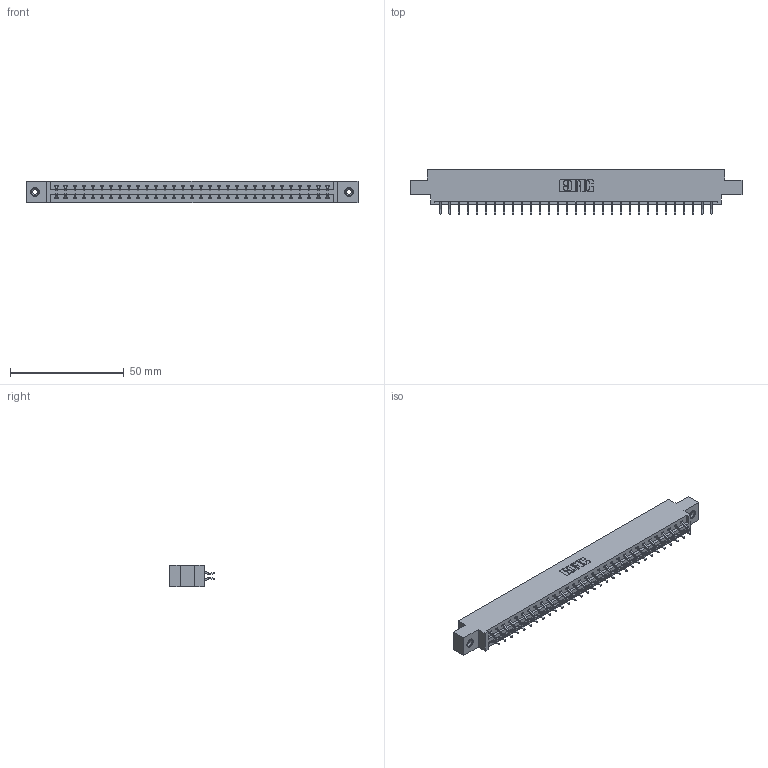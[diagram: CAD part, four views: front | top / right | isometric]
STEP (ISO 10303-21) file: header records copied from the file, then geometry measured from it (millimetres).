
FILE_DESCRIPTION (( 'STEP AP203' ), '1' );
FILE_NAME ('387-062-556-808.STEP', '2018-09-21T06:06:02', ( '' ), ( '' ), 'SwSTEP 2.0', 'SolidWorks 2016', '' );
FILE_SCHEMA (( 'CONFIG_CONTROL_DESIGN' ));
Length unit declared in the file: inch
Products named in the file (4): 345-250-001_345-250-003-102; 387-062-556-808; 337 Part_0.170 Offset - 0.156 Dia-TI; 345-292-001_556 Tail
Assembly tree (65 placements, depth 2):
  387-062-556-808
    337 Part_0.170 Offset - 0.156 Dia-TI
    345-292-001_556 Tail  x62
    345-250-001_345-250-003-102  x2
Bounding box: 145.85 x 19.57 x 9.4 mm (x, y, z)
Volume: 15097.6 mm3; surface area: 17027.4 mm2
Topology: 65 solids, 65 shells, 3898 faces, 11557 edges, 7614 vertices
Faces by surface type: plane 2710, cylinder 1172, cone 12, torus 4
Entity records: 26996 total; most frequent: CARTESIAN_POINT 4553, ORIENTED_EDGE 4470, DIRECTION 3913, EDGE_CURVE 2235, LINE 2079, VECTOR 2079, VERTEX_POINT 1484, AXIS2_PLACEMENT_3D 917
